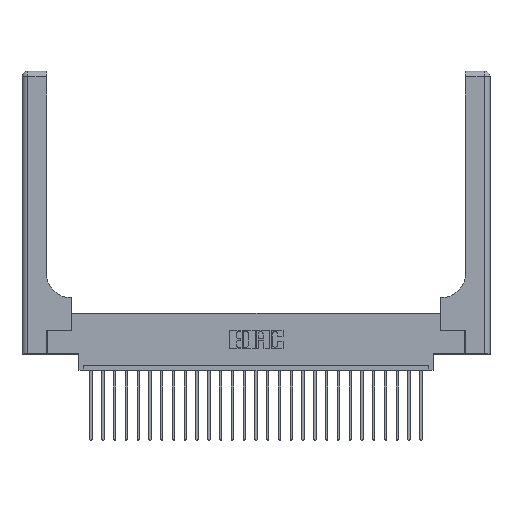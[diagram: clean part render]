
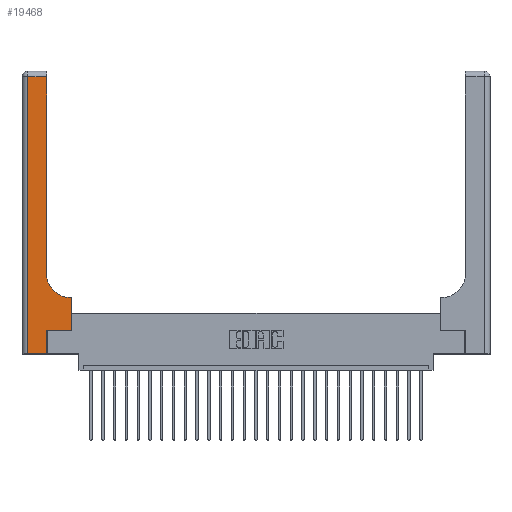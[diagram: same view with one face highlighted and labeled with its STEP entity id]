
A CAD part, top view. The second image highlights one B-rep face of the part: STEP entity #19468.
In plain terms, the highlighted planar face has unit normal (0, 0, 1).
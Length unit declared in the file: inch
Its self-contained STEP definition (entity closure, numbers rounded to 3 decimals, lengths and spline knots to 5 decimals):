
#333 = DIRECTION ( 'NONE',  ( 0., 1., 0. ) ) ;
#518 = CARTESIAN_POINT ( 'NONE',  ( 0.265, 0., 0.37 ) ) ;
#660 = CARTESIAN_POINT ( 'NONE',  ( 0.528, 0.6, 0.37 ) ) ;
#942 = VERTEX_POINT ( 'NONE', #22531 ) ;
#1058 = DIRECTION ( 'NONE',  ( -1., 0., 0. ) ) ;
#1840 = CARTESIAN_POINT ( 'NONE',  ( 0.26, 0.85, 0.37 ) ) ;
#2094 = VERTEX_POINT ( 'NONE', #17044 ) ;
#2493 = LINE ( 'NONE', #7271, #3677 ) ;
#3296 = VERTEX_POINT ( 'NONE', #20534 ) ;
#3677 = VECTOR ( 'NONE', #5322, 39.37008 ) ;
#3802 = DIRECTION ( 'NONE',  ( 0., 1., 0. ) ) ;
#4074 = CARTESIAN_POINT ( 'NONE',  ( 0., 2.94, 0.37 ) ) ;
#4409 = FACE_OUTER_BOUND ( 'NONE', #22327, .T. ) ;
#4657 = VECTOR ( 'NONE', #6145, 39.37008 ) ;
#5225 = VECTOR ( 'NONE', #6095, 39.37008 ) ;
#5322 = DIRECTION ( 'NONE',  ( 1., 0., 0. ) ) ;
#5512 = DIRECTION ( 'NONE',  ( 0., 0., -1. ) ) ;
#6095 = DIRECTION ( 'NONE',  ( -1., 0., 0. ) ) ;
#6145 = DIRECTION ( 'NONE',  ( 0., 1., 0. ) ) ;
#6436 = LINE ( 'NONE', #4074, #5225 ) ;
#6502 = DIRECTION ( 'NONE',  ( 0., -1., 0. ) ) ;
#6512 = LINE ( 'NONE', #15612, #13708 ) ;
#7151 = LINE ( 'NONE', #7181, #10821 ) ;
#7181 = CARTESIAN_POINT ( 'NONE',  ( 0., 0., 0.37 ) ) ;
#7271 = CARTESIAN_POINT ( 'NONE',  ( 0.265, 0.25, 0.37 ) ) ;
#7525 = CARTESIAN_POINT ( 'NONE',  ( 0.51, 0.85, 0.37 ) ) ;
#8096 = CARTESIAN_POINT ( 'NONE',  ( 0.26, 3., 0.37 ) ) ;
#8120 = ORIENTED_EDGE ( 'NONE', *, *, #18444, .T. ) ;
#8178 = EDGE_CURVE ( 'NONE', #9714, #20037, #17462, .T. ) ;
#9082 = ORIENTED_EDGE ( 'NONE', *, *, #24833, .T. ) ;
#9552 = AXIS2_PLACEMENT_3D ( 'NONE', #7525, #5512, #11324 ) ;
#9714 = VERTEX_POINT ( 'NONE', #660 ) ;
#9763 = CIRCLE ( 'NONE', #9552, 0.25 ) ;
#9811 = CARTESIAN_POINT ( 'NONE',  ( 0., 3., 0.37 ) ) ;
#10011 = ORIENTED_EDGE ( 'NONE', *, *, #12740, .T. ) ;
#10218 = ORIENTED_EDGE ( 'NONE', *, *, #24625, .T. ) ;
#10596 = VERTEX_POINT ( 'NONE', #18932 ) ;
#10821 = VECTOR ( 'NONE', #16584, 39.37008 ) ;
#10940 = ORIENTED_EDGE ( 'NONE', *, *, #14421, .T. ) ;
#11324 = DIRECTION ( 'NONE',  ( 1., 0., 0. ) ) ;
#11720 = DIRECTION ( 'NONE',  ( -1., 0., 0. ) ) ;
#12438 = VERTEX_POINT ( 'NONE', #1840 ) ;
#12740 = EDGE_CURVE ( 'NONE', #20037, #12438, #9763, .T. ) ;
#12766 = LINE ( 'NONE', #22112, #17297 ) ;
#12798 = VERTEX_POINT ( 'NONE', #518 ) ;
#13708 = VECTOR ( 'NONE', #333, 39.37008 ) ;
#14421 = EDGE_CURVE ( 'NONE', #12438, #10596, #16161, .T. ) ;
#15190 = LINE ( 'NONE', #15393, #17017 ) ;
#15393 = CARTESIAN_POINT ( 'NONE',  ( 0.528, 0.25, 0.37 ) ) ;
#15502 = EDGE_CURVE ( 'NONE', #3296, #2094, #2493, .T. ) ;
#15543 = PLANE ( 'NONE',  #20846 ) ;
#15612 = CARTESIAN_POINT ( 'NONE',  ( 0.265, 0., 0.37 ) ) ;
#16161 = LINE ( 'NONE', #8096, #4657 ) ;
#16281 = VECTOR ( 'NONE', #1058, 39.37008 ) ;
#16530 = CARTESIAN_POINT ( 'NONE',  ( 0.51, 0.6, 0.37 ) ) ;
#16584 = DIRECTION ( 'NONE',  ( 1., 0., 0. ) ) ;
#17017 = VECTOR ( 'NONE', #3802, 39.37008 ) ;
#17044 = CARTESIAN_POINT ( 'NONE',  ( 0.528, 0.25, 0.37 ) ) ;
#17297 = VECTOR ( 'NONE', #6502, 39.37008 ) ;
#17462 = LINE ( 'NONE', #24350, #16281 ) ;
#18444 = EDGE_CURVE ( 'NONE', #24517, #12798, #7151, .T. ) ;
#18932 = CARTESIAN_POINT ( 'NONE',  ( 0.26, 2.94, 0.37 ) ) ;
#19345 = ORIENTED_EDGE ( 'NONE', *, *, #15502, .T. ) ;
#19468 = ADVANCED_FACE ( 'NONE', ( #4409 ), #15543, .F. ) ;
#20037 = VERTEX_POINT ( 'NONE', #16530 ) ;
#20534 = CARTESIAN_POINT ( 'NONE',  ( 0.265, 0.25, 0.37 ) ) ;
#20652 = ORIENTED_EDGE ( 'NONE', *, *, #22969, .T. ) ;
#20846 = AXIS2_PLACEMENT_3D ( 'NONE', #9811, #23375, #11720 ) ;
#21254 = CARTESIAN_POINT ( 'NONE',  ( 0.06, 0., 0.37 ) ) ;
#22112 = CARTESIAN_POINT ( 'NONE',  ( 0.06, 3., 0.37 ) ) ;
#22194 = ORIENTED_EDGE ( 'NONE', *, *, #8178, .T. ) ;
#22327 = EDGE_LOOP ( 'NONE', ( #10940, #10218, #9082, #8120, #20652, #19345, #25022, #22194, #10011 ) ) ;
#22531 = CARTESIAN_POINT ( 'NONE',  ( 0.06, 2.94, 0.37 ) ) ;
#22969 = EDGE_CURVE ( 'NONE', #12798, #3296, #6512, .T. ) ;
#23375 = DIRECTION ( 'NONE',  ( 0., 0., -1. ) ) ;
#24350 = CARTESIAN_POINT ( 'NONE',  ( 0.26, 0.6, 0.37 ) ) ;
#24517 = VERTEX_POINT ( 'NONE', #21254 ) ;
#24552 = EDGE_CURVE ( 'NONE', #2094, #9714, #15190, .T. ) ;
#24625 = EDGE_CURVE ( 'NONE', #10596, #942, #6436, .T. ) ;
#24833 = EDGE_CURVE ( 'NONE', #942, #24517, #12766, .T. ) ;
#25022 = ORIENTED_EDGE ( 'NONE', *, *, #24552, .T. ) ;
